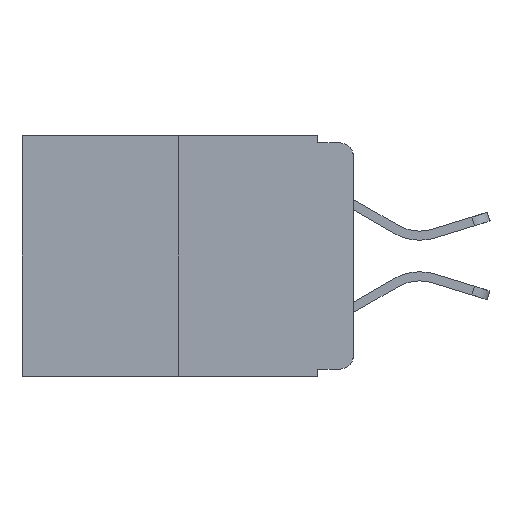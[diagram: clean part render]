
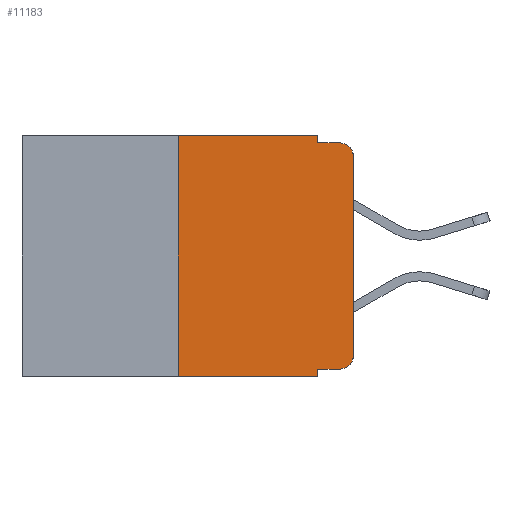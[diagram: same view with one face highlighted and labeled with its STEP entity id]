
A CAD part, left-side view. The second image highlights one B-rep face of the part: STEP entity #11183.
In plain terms, the highlighted planar face has unit normal (-1, 0, 0).
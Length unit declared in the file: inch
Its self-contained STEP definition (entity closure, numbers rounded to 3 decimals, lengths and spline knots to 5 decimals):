
#4 = LINE ( 'NONE', #4367, #11019 ) ;
#121 = ORIENTED_EDGE ( 'NONE', *, *, #5608, .T. ) ;
#471 = EDGE_CURVE ( 'NONE', #8224, #3848, #10363, .T. ) ;
#581 = CARTESIAN_POINT ( 'NONE',  ( 0., 0.473, 0. ) ) ;
#721 = DIRECTION ( 'NONE',  ( 0., 0., -1. ) ) ;
#735 = VERTEX_POINT ( 'NONE', #8203 ) ;
#742 = CARTESIAN_POINT ( 'NONE',  ( 0., 0.473, 0. ) ) ;
#780 = CARTESIAN_POINT ( 'NONE',  ( 0., 0.25, 0. ) ) ;
#1000 = VECTOR ( 'NONE', #1080, 39.37008 ) ;
#1080 = DIRECTION ( 'NONE',  ( 0., 0., 1. ) ) ;
#1121 = DIRECTION ( 'NONE',  ( 0., -1., 0. ) ) ;
#1198 = EDGE_CURVE ( 'NONE', #1722, #5156, #7170, .T. ) ;
#1665 = DIRECTION ( 'NONE',  ( 0., 0., -1. ) ) ;
#1722 = VERTEX_POINT ( 'NONE', #1762 ) ;
#1739 = EDGE_LOOP ( 'NONE', ( #5730, #3857, #1955, #3336, #4370, #2802, #11280, #9846, #8459, #121 ) ) ;
#1762 = CARTESIAN_POINT ( 'NONE',  ( 0., 0.25, -0.343 ) ) ;
#1763 = VERTEX_POINT ( 'NONE', #4053 ) ;
#1851 = VECTOR ( 'NONE', #721, 39.37008 ) ;
#1955 = ORIENTED_EDGE ( 'NONE', *, *, #12800, .F. ) ;
#2074 = CARTESIAN_POINT ( 'NONE',  ( 0., 0.051, 0. ) ) ;
#2081 = CIRCLE ( 'NONE', #11063, 0.02 ) ;
#2628 = CARTESIAN_POINT ( 'NONE',  ( 0., 0.051, -0.01 ) ) ;
#2629 = EDGE_CURVE ( 'NONE', #5508, #5826, #6302, .T. ) ;
#2802 = ORIENTED_EDGE ( 'NONE', *, *, #1198, .F. ) ;
#3285 = CIRCLE ( 'NONE', #10585, 0.02 ) ;
#3336 = ORIENTED_EDGE ( 'NONE', *, *, #471, .F. ) ;
#3374 = DIRECTION ( 'NONE',  ( -1., 0., 0. ) ) ;
#3641 = VERTEX_POINT ( 'NONE', #11849 ) ;
#3793 = CARTESIAN_POINT ( 'NONE',  ( 0., 0., -0.313 ) ) ;
#3833 = VECTOR ( 'NONE', #6310, 39.37008 ) ;
#3848 = VERTEX_POINT ( 'NONE', #2628 ) ;
#3857 = ORIENTED_EDGE ( 'NONE', *, *, #12128, .T. ) ;
#4053 = CARTESIAN_POINT ( 'NONE',  ( 0., 0., -0.03 ) ) ;
#4256 = LINE ( 'NONE', #742, #6840 ) ;
#4367 = CARTESIAN_POINT ( 'NONE',  ( 0., 0.473, -0.343 ) ) ;
#4370 = ORIENTED_EDGE ( 'NONE', *, *, #12487, .F. ) ;
#4827 = AXIS2_PLACEMENT_3D ( 'NONE', #581, #8191, #1665 ) ;
#4854 = EDGE_CURVE ( 'NONE', #5508, #3641, #12207, .T. ) ;
#5156 = VERTEX_POINT ( 'NONE', #7879 ) ;
#5191 = CARTESIAN_POINT ( 'NONE',  ( 0., 0.051, -0.333 ) ) ;
#5204 = LINE ( 'NONE', #5473, #8063 ) ;
#5250 = CARTESIAN_POINT ( 'NONE',  ( 0., 0.051, 0. ) ) ;
#5324 = CARTESIAN_POINT ( 'NONE',  ( 0., 0.02, -0.313 ) ) ;
#5473 = CARTESIAN_POINT ( 'NONE',  ( 0., 0., 0. ) ) ;
#5508 = VERTEX_POINT ( 'NONE', #10382 ) ;
#5608 = EDGE_CURVE ( 'NONE', #3641, #8656, #3285, .T. ) ;
#5714 = FACE_OUTER_BOUND ( 'NONE', #1739, .T. ) ;
#5730 = ORIENTED_EDGE ( 'NONE', *, *, #11435, .T. ) ;
#5826 = VERTEX_POINT ( 'NONE', #5882 ) ;
#5882 = CARTESIAN_POINT ( 'NONE',  ( 0., 0.051, -0.343 ) ) ;
#6302 = LINE ( 'NONE', #6469, #11117 ) ;
#6310 = DIRECTION ( 'NONE',  ( 0., -1., 0. ) ) ;
#6427 = DIRECTION ( 'NONE',  ( 0., 0., -1. ) ) ;
#6469 = CARTESIAN_POINT ( 'NONE',  ( 0., 0.051, 0. ) ) ;
#6568 = DIRECTION ( 'NONE',  ( 0., 0., 1. ) ) ;
#6799 = DIRECTION ( 'NONE',  ( 0., 0., -1. ) ) ;
#6820 = CARTESIAN_POINT ( 'NONE',  ( 0., 0.051, -0.01 ) ) ;
#6840 = VECTOR ( 'NONE', #13396, 39.37008 ) ;
#6895 = EDGE_CURVE ( 'NONE', #1722, #5826, #4, .T. ) ;
#7170 = LINE ( 'NONE', #780, #1000 ) ;
#7878 = DIRECTION ( 'NONE',  ( 0., -1., 0. ) ) ;
#7879 = CARTESIAN_POINT ( 'NONE',  ( 0., 0.25, 0. ) ) ;
#8063 = VECTOR ( 'NONE', #6568, 39.37008 ) ;
#8140 = VECTOR ( 'NONE', #7878, 39.37008 ) ;
#8191 = DIRECTION ( 'NONE',  ( 1., 0., 0. ) ) ;
#8203 = CARTESIAN_POINT ( 'NONE',  ( 0., 0.02, -0.01 ) ) ;
#8224 = VERTEX_POINT ( 'NONE', #5250 ) ;
#8459 = ORIENTED_EDGE ( 'NONE', *, *, #4854, .T. ) ;
#8656 = VERTEX_POINT ( 'NONE', #3793 ) ;
#9742 = CARTESIAN_POINT ( 'NONE',  ( 0., 0.02, -0.03 ) ) ;
#9846 = ORIENTED_EDGE ( 'NONE', *, *, #2629, .F. ) ;
#10363 = LINE ( 'NONE', #2074, #1851 ) ;
#10382 = CARTESIAN_POINT ( 'NONE',  ( 0., 0.051, -0.333 ) ) ;
#10585 = AXIS2_PLACEMENT_3D ( 'NONE', #5324, #12595, #6427 ) ;
#10757 = DIRECTION ( 'NONE',  ( 0., 0., -1. ) ) ;
#11019 = VECTOR ( 'NONE', #1121, 39.37008 ) ;
#11063 = AXIS2_PLACEMENT_3D ( 'NONE', #9742, #3374, #10757 ) ;
#11117 = VECTOR ( 'NONE', #6799, 39.37008 ) ;
#11141 = LINE ( 'NONE', #6820, #8140 ) ;
#11183 = ADVANCED_FACE ( 'NONE', ( #5714 ), #12242, .F. ) ;
#11280 = ORIENTED_EDGE ( 'NONE', *, *, #6895, .T. ) ;
#11435 = EDGE_CURVE ( 'NONE', #8656, #1763, #5204, .T. ) ;
#11849 = CARTESIAN_POINT ( 'NONE',  ( 0., 0.02, -0.333 ) ) ;
#12128 = EDGE_CURVE ( 'NONE', #1763, #735, #2081, .T. ) ;
#12207 = LINE ( 'NONE', #5191, #3833 ) ;
#12242 = PLANE ( 'NONE',  #4827 ) ;
#12487 = EDGE_CURVE ( 'NONE', #5156, #8224, #4256, .T. ) ;
#12595 = DIRECTION ( 'NONE',  ( -1., 0., 0. ) ) ;
#12800 = EDGE_CURVE ( 'NONE', #3848, #735, #11141, .T. ) ;
#13396 = DIRECTION ( 'NONE',  ( 0., -1., 0. ) ) ;
